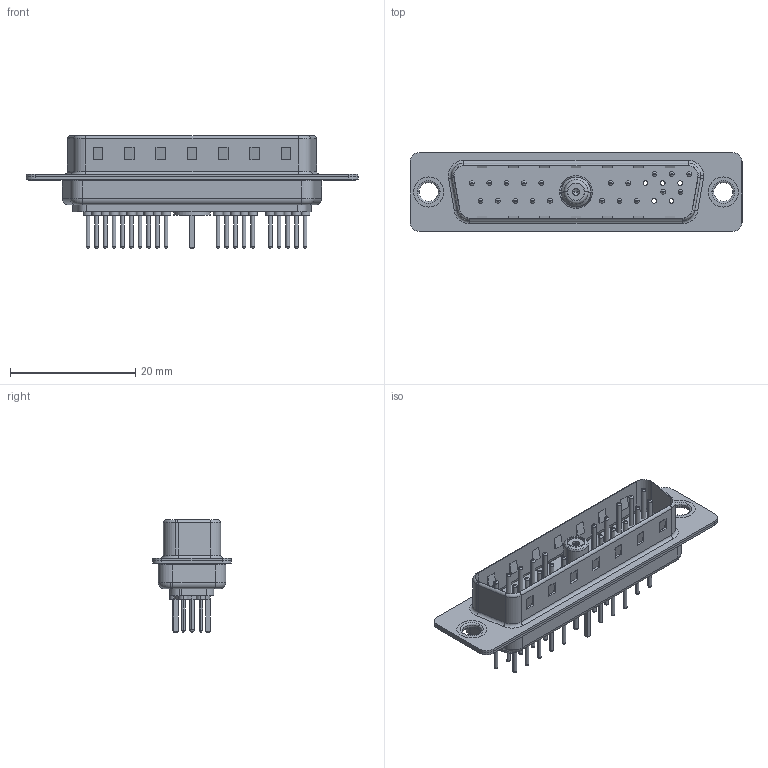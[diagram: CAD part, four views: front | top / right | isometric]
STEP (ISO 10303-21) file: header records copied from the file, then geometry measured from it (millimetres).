
FILE_DESCRIPTION (( 'STEP AP203' ), '1' );
FILE_NAME ('627-21W1624-7T1.STEP', '2019-05-28T02:40:22', ( '' ), ( '' ), 'SwSTEP 2.0', 'SolidWorks 2016', '' );
FILE_SCHEMA (( 'CONFIG_CONTROL_DESIGN' ));
Length unit declared in the file: millimetre
Products named in the file (13): 627-21W1624-7T1; Insulator Socket; 627Combo Shell Rear_25 Contacts; 627Combo Contact Row 2_24; 627Combo Thru Hole Rivet; Locking Collar; Socket_Str; 627Combo Housing_21W1; 627Combo Shell Front_25 Contacts; Co-Ax Jack Assy_S; Insulator Socket 2; 627Combo Contact Row 1_24; Co-Ax Jack_Straight PC Tail
Assembly tree (31 placements, depth 3):
  627-21W1624-7T1
    627Combo Housing_21W1
    627Combo Shell Rear_25 Contacts
    627Combo Shell Front_25 Contacts
    627Combo Thru Hole Rivet  x2
    Co-Ax Jack Assy_S
      Co-Ax Jack_Straight PC Tail
      Insulator Socket
      Insulator Socket 2
      Locking Collar
      Socket_Str
    627Combo Contact Row 1_24  x10
    627Combo Contact Row 2_24  x10
Bounding box: 53 x 12.6 x 17.9 mm (x, y, z)
Volume: 2662.2 mm3; surface area: 7086.8 mm2
Topology: 30 solids, 30 shells, 1201 faces, 2604 edges, 1582 vertices
Faces by surface type: cylinder 448, torus 382, plane 358, cone 9, bspline 2, sphere 2
Entity records: 21294 total; most frequent: DIRECTION 3656, CARTESIAN_POINT 3374, ORIENTED_EDGE 3100, EDGE_CURVE 1550, AXIS2_PLACEMENT_3D 1441, VERTEX_POINT 982, EDGE_LOOP 818, VECTOR 774
